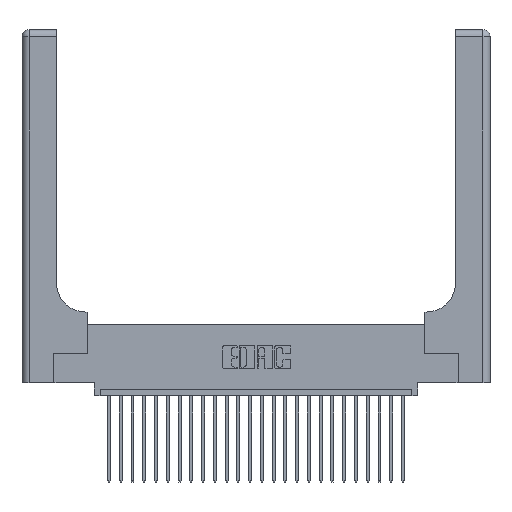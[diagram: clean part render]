
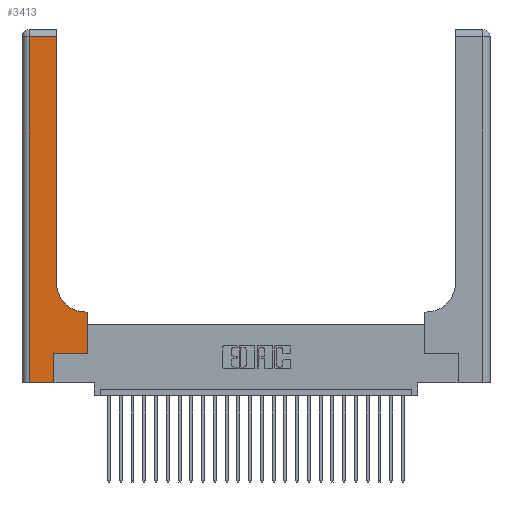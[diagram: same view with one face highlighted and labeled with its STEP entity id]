
A CAD part, top view. The second image highlights one B-rep face of the part: STEP entity #3413.
In plain terms, the highlighted planar face has unit normal (0, 0, 1).
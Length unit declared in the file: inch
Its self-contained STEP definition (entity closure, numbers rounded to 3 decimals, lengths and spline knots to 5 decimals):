
#22 = CARTESIAN_POINT ( 'NONE',  ( 0.2915, 3., 0.37 ) ) ;
#382 = EDGE_CURVE ( 'NONE', #7296, #7126, #6729, .T. ) ;
#691 = CARTESIAN_POINT ( 'NONE',  ( 0.5585, 0.25, 0.37 ) ) ;
#876 = PLANE ( 'NONE',  #14685 ) ;
#914 = FACE_OUTER_BOUND ( 'NONE', #8439, .T. ) ;
#1240 = VECTOR ( 'NONE', #26700, 39.37008 ) ;
#1762 = DIRECTION ( 'NONE',  ( 0., 1., 0. ) ) ;
#2613 = EDGE_CURVE ( 'NONE', #12732, #8394, #25422, .T. ) ;
#2860 = DIRECTION ( 'NONE',  ( 1., 0., 0. ) ) ;
#2881 = DIRECTION ( 'NONE',  ( 0., 0., -1. ) ) ;
#3413 = ADVANCED_FACE ( 'NONE', ( #914 ), #876, .F. ) ;
#3536 = ORIENTED_EDGE ( 'NONE', *, *, #4245, .T. ) ;
#3803 = LINE ( 'NONE', #11160, #20756 ) ;
#3937 = CARTESIAN_POINT ( 'NONE',  ( 0.2915, 0.85, 0.37 ) ) ;
#3942 = VECTOR ( 'NONE', #16441, 39.37008 ) ;
#4027 = CARTESIAN_POINT ( 'NONE',  ( 0., 0., 0.37 ) ) ;
#4150 = CARTESIAN_POINT ( 'NONE',  ( 0., 2.94, 0.37 ) ) ;
#4245 = EDGE_CURVE ( 'NONE', #21248, #19197, #18462, .T. ) ;
#4993 = CARTESIAN_POINT ( 'NONE',  ( 0.06, 2.94, 0.37 ) ) ;
#5109 = CARTESIAN_POINT ( 'NONE',  ( 0.06, 0., 0.37 ) ) ;
#5834 = ORIENTED_EDGE ( 'NONE', *, *, #16019, .T. ) ;
#6400 = VERTEX_POINT ( 'NONE', #10094 ) ;
#6729 = LINE ( 'NONE', #4150, #18473 ) ;
#7012 = CARTESIAN_POINT ( 'NONE',  ( 0.5585, 0.6, 0.37 ) ) ;
#7100 = DIRECTION ( 'NONE',  ( 0., -1., 0. ) ) ;
#7126 = VERTEX_POINT ( 'NONE', #4993 ) ;
#7296 = VERTEX_POINT ( 'NONE', #18075 ) ;
#7731 = DIRECTION ( 'NONE',  ( 0., 0., -1. ) ) ;
#8394 = VERTEX_POINT ( 'NONE', #7012 ) ;
#8439 = EDGE_LOOP ( 'NONE', ( #8578, #26180, #15260, #11658, #21832, #5834, #23841, #23320, #3536 ) ) ;
#8578 = ORIENTED_EDGE ( 'NONE', *, *, #26681, .T. ) ;
#9383 = VECTOR ( 'NONE', #21066, 39.37008 ) ;
#9833 = EDGE_CURVE ( 'NONE', #8394, #21248, #17556, .T. ) ;
#10094 = CARTESIAN_POINT ( 'NONE',  ( 0.269, 0.25, 0.37 ) ) ;
#10772 = CARTESIAN_POINT ( 'NONE',  ( 0.2915, 0.6, 0.37 ) ) ;
#11160 = CARTESIAN_POINT ( 'NONE',  ( 0.269, 0.25, 0.37 ) ) ;
#11658 = ORIENTED_EDGE ( 'NONE', *, *, #19248, .T. ) ;
#12378 = LINE ( 'NONE', #15569, #13716 ) ;
#12732 = VERTEX_POINT ( 'NONE', #691 ) ;
#13046 = LINE ( 'NONE', #22, #18915 ) ;
#13471 = VECTOR ( 'NONE', #7100, 39.37008 ) ;
#13716 = VECTOR ( 'NONE', #19745, 39.37008 ) ;
#13839 = CARTESIAN_POINT ( 'NONE',  ( 0., 3., 0.37 ) ) ;
#14685 = AXIS2_PLACEMENT_3D ( 'NONE', #13839, #7731, #24404 ) ;
#15091 = LINE ( 'NONE', #26080, #13471 ) ;
#15260 = ORIENTED_EDGE ( 'NONE', *, *, #18368, .T. ) ;
#15563 = DIRECTION ( 'NONE',  ( -1., 0., 0. ) ) ;
#15569 = CARTESIAN_POINT ( 'NONE',  ( 0.269, 0., 0.37 ) ) ;
#15834 = CARTESIAN_POINT ( 'NONE',  ( 0.5415, 0.6, 0.37 ) ) ;
#16019 = EDGE_CURVE ( 'NONE', #6400, #12732, #3803, .T. ) ;
#16441 = DIRECTION ( 'NONE',  ( 1., 0., 0. ) ) ;
#17248 = CARTESIAN_POINT ( 'NONE',  ( 0.269, 0., 0.37 ) ) ;
#17556 = LINE ( 'NONE', #10772, #9383 ) ;
#18075 = CARTESIAN_POINT ( 'NONE',  ( 0.2915, 2.94, 0.37 ) ) ;
#18348 = AXIS2_PLACEMENT_3D ( 'NONE', #23585, #2881, #26057 ) ;
#18368 = EDGE_CURVE ( 'NONE', #7126, #19615, #15091, .T. ) ;
#18462 = CIRCLE ( 'NONE', #18348, 0.25 ) ;
#18473 = VECTOR ( 'NONE', #15563, 39.37008 ) ;
#18915 = VECTOR ( 'NONE', #1762, 39.37008 ) ;
#19197 = VERTEX_POINT ( 'NONE', #3937 ) ;
#19248 = EDGE_CURVE ( 'NONE', #19615, #19355, #22852, .T. ) ;
#19355 = VERTEX_POINT ( 'NONE', #17248 ) ;
#19615 = VERTEX_POINT ( 'NONE', #5109 ) ;
#19745 = DIRECTION ( 'NONE',  ( 0., 1., 0. ) ) ;
#20756 = VECTOR ( 'NONE', #2860, 39.37008 ) ;
#21066 = DIRECTION ( 'NONE',  ( -1., 0., 0. ) ) ;
#21248 = VERTEX_POINT ( 'NONE', #15834 ) ;
#21832 = ORIENTED_EDGE ( 'NONE', *, *, #26483, .T. ) ;
#22852 = LINE ( 'NONE', #4027, #3942 ) ;
#23320 = ORIENTED_EDGE ( 'NONE', *, *, #9833, .T. ) ;
#23585 = CARTESIAN_POINT ( 'NONE',  ( 0.5415, 0.85, 0.37 ) ) ;
#23841 = ORIENTED_EDGE ( 'NONE', *, *, #2613, .T. ) ;
#24404 = DIRECTION ( 'NONE',  ( -1., 0., 0. ) ) ;
#24756 = CARTESIAN_POINT ( 'NONE',  ( 0.5585, 0.25, 0.37 ) ) ;
#25422 = LINE ( 'NONE', #24756, #1240 ) ;
#26057 = DIRECTION ( 'NONE',  ( 1., 0., 0. ) ) ;
#26080 = CARTESIAN_POINT ( 'NONE',  ( 0.06, 3., 0.37 ) ) ;
#26180 = ORIENTED_EDGE ( 'NONE', *, *, #382, .T. ) ;
#26483 = EDGE_CURVE ( 'NONE', #19355, #6400, #12378, .T. ) ;
#26681 = EDGE_CURVE ( 'NONE', #19197, #7296, #13046, .T. ) ;
#26700 = DIRECTION ( 'NONE',  ( 0., 1., 0. ) ) ;
